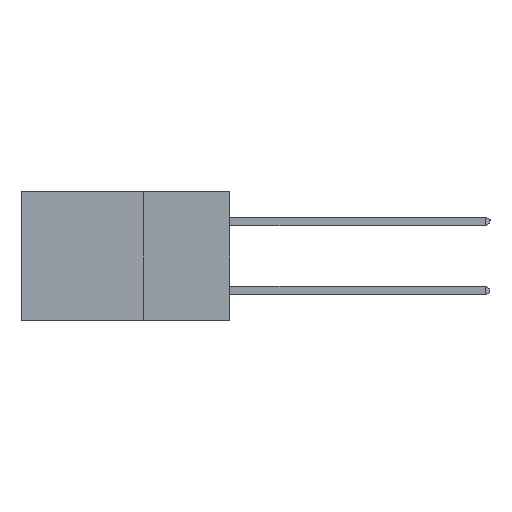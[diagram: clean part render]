
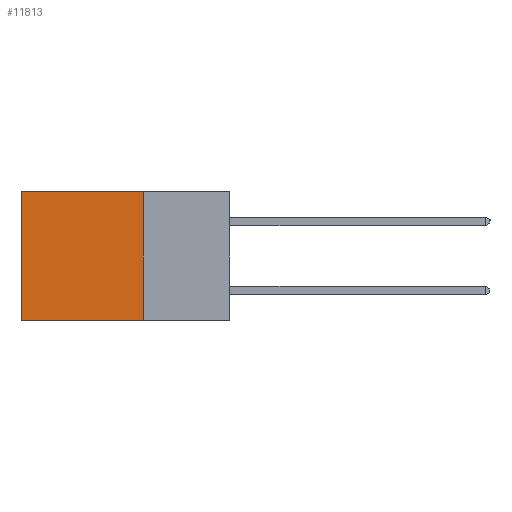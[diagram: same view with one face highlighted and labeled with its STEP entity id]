
A CAD part, left-side view. The second image highlights one B-rep face of the part: STEP entity #11813.
In plain terms, the highlighted planar face has unit normal (-1, 0, 0).
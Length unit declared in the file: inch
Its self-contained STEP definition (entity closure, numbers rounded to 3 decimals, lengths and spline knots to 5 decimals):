
#330 = FACE_OUTER_BOUND ( 'NONE', #5555, .T. ) ;
#1522 = CARTESIAN_POINT ( 'NONE',  ( 0.2615, 0.25, -0.37 ) ) ;
#1590 = VERTEX_POINT ( 'NONE', #7141 ) ;
#1648 = EDGE_CURVE ( 'NONE', #1590, #10481, #5009, .T. ) ;
#1764 = CARTESIAN_POINT ( 'NONE',  ( 0.2615, 0.25, 0. ) ) ;
#1778 = CARTESIAN_POINT ( 'NONE',  ( 0.2615, 0.25, -0.37 ) ) ;
#2202 = LINE ( 'NONE', #11608, #3157 ) ;
#2784 = DIRECTION ( 'NONE',  ( 1., 0., 0. ) ) ;
#2906 = VERTEX_POINT ( 'NONE', #13750 ) ;
#3157 = VECTOR ( 'NONE', #8011, 39.37008 ) ;
#3768 = ORIENTED_EDGE ( 'NONE', *, *, #1648, .F. ) ;
#3886 = DIRECTION ( 'NONE',  ( 0., 1., 0. ) ) ;
#4678 = ORIENTED_EDGE ( 'NONE', *, *, #13641, .T. ) ;
#5009 = LINE ( 'NONE', #7300, #10423 ) ;
#5166 = CARTESIAN_POINT ( 'NONE',  ( 0.2615, 0.6, -0.37 ) ) ;
#5531 = DIRECTION ( 'NONE',  ( 0., 0., -1. ) ) ;
#5555 = EDGE_LOOP ( 'NONE', ( #4678, #3768, #8774, #14251 ) ) ;
#7141 = CARTESIAN_POINT ( 'NONE',  ( 0.2615, 0.25, -0.37 ) ) ;
#7300 = CARTESIAN_POINT ( 'NONE',  ( 0.2615, 0.25, -0.37 ) ) ;
#7407 = VECTOR ( 'NONE', #5531, 39.37008 ) ;
#8011 = DIRECTION ( 'NONE',  ( 0., 0., -1. ) ) ;
#8690 = AXIS2_PLACEMENT_3D ( 'NONE', #1522, #2784, #9069 ) ;
#8774 = ORIENTED_EDGE ( 'NONE', *, *, #11324, .F. ) ;
#9069 = DIRECTION ( 'NONE',  ( 0., 0., -1. ) ) ;
#10423 = VECTOR ( 'NONE', #3886, 39.37008 ) ;
#10481 = VERTEX_POINT ( 'NONE', #5166 ) ;
#11324 = EDGE_CURVE ( 'NONE', #14660, #1590, #11567, .T. ) ;
#11567 = LINE ( 'NONE', #1778, #7407 ) ;
#11608 = CARTESIAN_POINT ( 'NONE',  ( 0.2615, 0.6, -0.37 ) ) ;
#11813 = ADVANCED_FACE ( 'NONE', ( #330 ), #12668, .F. ) ;
#12597 = LINE ( 'NONE', #1764, #14587 ) ;
#12668 = PLANE ( 'NONE',  #8690 ) ;
#13024 = EDGE_CURVE ( 'NONE', #14660, #2906, #12597, .T. ) ;
#13465 = CARTESIAN_POINT ( 'NONE',  ( 0.2615, 0.25, 0. ) ) ;
#13641 = EDGE_CURVE ( 'NONE', #2906, #10481, #2202, .T. ) ;
#13750 = CARTESIAN_POINT ( 'NONE',  ( 0.2615, 0.6, 0. ) ) ;
#14251 = ORIENTED_EDGE ( 'NONE', *, *, #13024, .T. ) ;
#14587 = VECTOR ( 'NONE', #15134, 39.37008 ) ;
#14660 = VERTEX_POINT ( 'NONE', #13465 ) ;
#15134 = DIRECTION ( 'NONE',  ( 0., 1., 0. ) ) ;
